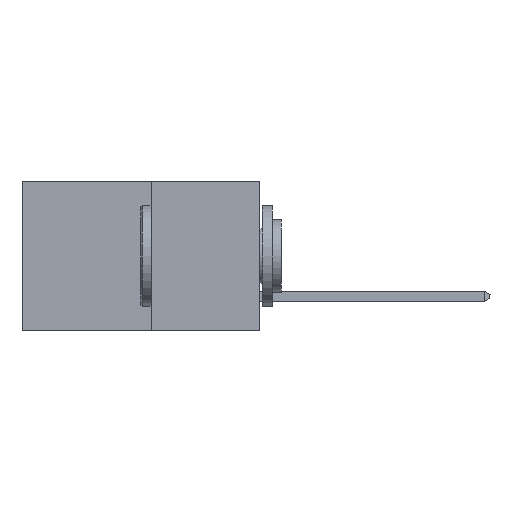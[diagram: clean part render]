
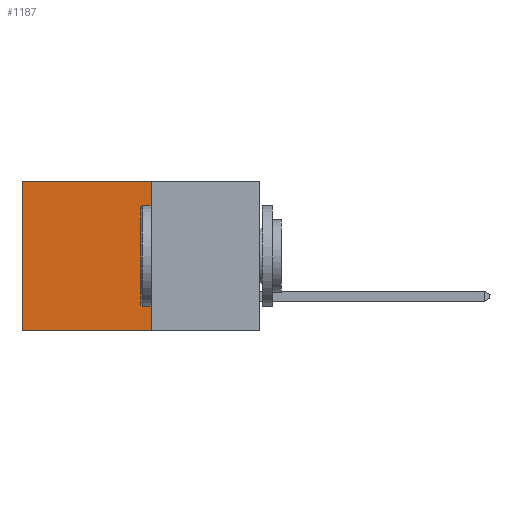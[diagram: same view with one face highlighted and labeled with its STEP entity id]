
A CAD part, left-side view. The second image highlights one B-rep face of the part: STEP entity #1187.
In plain terms, the highlighted planar face has unit normal (-1, 0, 0).
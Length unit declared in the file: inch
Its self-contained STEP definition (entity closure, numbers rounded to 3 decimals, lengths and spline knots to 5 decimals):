
#104 = FACE_OUTER_BOUND ( 'NONE', #6420, .T. ) ;
#262 = LINE ( 'NONE', #4557, #2056 ) ;
#584 = ORIENTED_EDGE ( 'NONE', *, *, #5732, .T. ) ;
#657 = LINE ( 'NONE', #8769, #4927 ) ;
#1187 = ADVANCED_FACE ( 'NONE', ( #104 ), #8375, .F. ) ;
#2016 = CARTESIAN_POINT ( 'NONE',  ( 0.277, 0.59, -0.37 ) ) ;
#2047 = DIRECTION ( 'NONE',  ( 0., 0., -1. ) ) ;
#2056 = VECTOR ( 'NONE', #2313, 39.37008 ) ;
#2313 = DIRECTION ( 'NONE',  ( 0., 0., -1. ) ) ;
#2727 = EDGE_CURVE ( 'NONE', #8728, #3554, #657, .T. ) ;
#3151 = VECTOR ( 'NONE', #4535, 39.37008 ) ;
#3554 = VERTEX_POINT ( 'NONE', #3781 ) ;
#3781 = CARTESIAN_POINT ( 'NONE',  ( 0.277, 0.27, -0.37 ) ) ;
#4535 = DIRECTION ( 'NONE',  ( 0., 1., 0. ) ) ;
#4557 = CARTESIAN_POINT ( 'NONE',  ( 0.277, 0.59, -0.37 ) ) ;
#4622 = ORIENTED_EDGE ( 'NONE', *, *, #2727, .F. ) ;
#4927 = VECTOR ( 'NONE', #9096, 39.37008 ) ;
#5108 = CARTESIAN_POINT ( 'NONE',  ( 0.277, 0.27, -0.37 ) ) ;
#5173 = LINE ( 'NONE', #8167, #8837 ) ;
#5244 = DIRECTION ( 'NONE',  ( 0., 1., 0. ) ) ;
#5428 = EDGE_CURVE ( 'NONE', #3554, #5475, #9237, .T. ) ;
#5475 = VERTEX_POINT ( 'NONE', #2016 ) ;
#5732 = EDGE_CURVE ( 'NONE', #7229, #5475, #262, .T. ) ;
#6420 = EDGE_LOOP ( 'NONE', ( #584, #9648, #4622, #8051 ) ) ;
#7168 = CARTESIAN_POINT ( 'NONE',  ( 0.277, 0.59, 0. ) ) ;
#7229 = VERTEX_POINT ( 'NONE', #7168 ) ;
#7416 = AXIS2_PLACEMENT_3D ( 'NONE', #9120, #7518, #2047 ) ;
#7518 = DIRECTION ( 'NONE',  ( 1., 0., 0. ) ) ;
#7586 = CARTESIAN_POINT ( 'NONE',  ( 0.277, 0.27, 0. ) ) ;
#8051 = ORIENTED_EDGE ( 'NONE', *, *, #8609, .T. ) ;
#8167 = CARTESIAN_POINT ( 'NONE',  ( 0.277, 0.27, 0. ) ) ;
#8375 = PLANE ( 'NONE',  #7416 ) ;
#8609 = EDGE_CURVE ( 'NONE', #8728, #7229, #5173, .T. ) ;
#8728 = VERTEX_POINT ( 'NONE', #7586 ) ;
#8769 = CARTESIAN_POINT ( 'NONE',  ( 0.277, 0.27, -0.37 ) ) ;
#8837 = VECTOR ( 'NONE', #5244, 39.37008 ) ;
#9096 = DIRECTION ( 'NONE',  ( 0., 0., -1. ) ) ;
#9120 = CARTESIAN_POINT ( 'NONE',  ( 0.277, 0.27, -0.37 ) ) ;
#9237 = LINE ( 'NONE', #5108, #3151 ) ;
#9648 = ORIENTED_EDGE ( 'NONE', *, *, #5428, .F. ) ;
